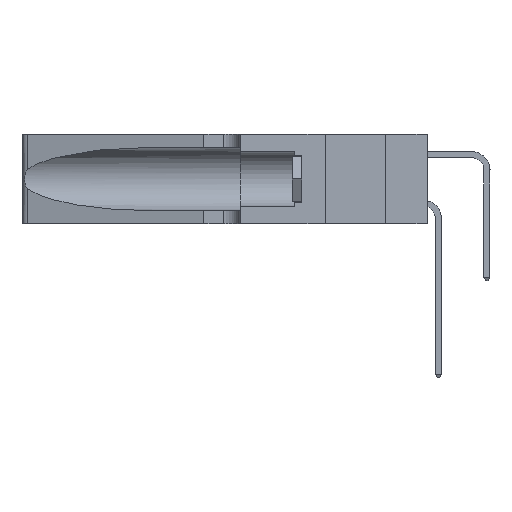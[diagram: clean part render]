
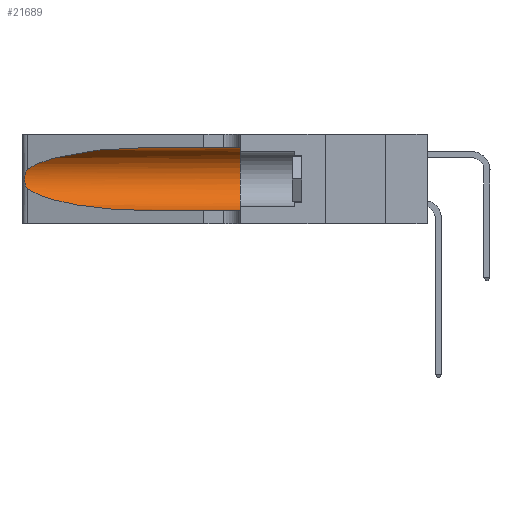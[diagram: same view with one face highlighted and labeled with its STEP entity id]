
A CAD part, left-side view. The second image highlights one B-rep face of the part: STEP entity #21689.
In plain terms, the highlighted cylindrical face has radius 3.308 mm (diameter 6.617 mm), a partial arc.
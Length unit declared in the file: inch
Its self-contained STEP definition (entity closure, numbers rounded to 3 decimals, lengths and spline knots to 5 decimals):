
#29 =( BOUNDED_CURVE ( )  B_SPLINE_CURVE ( 3, ( #14453, #12315, #16738, #3246 ),
 .UNSPECIFIED., .F., .T. ) 
 B_SPLINE_CURVE_WITH_KNOTS ( ( 4, 4 ),
 ( 1.5708, 2.84003 ),
 .UNSPECIFIED. ) 
 CURVE ( )  GEOMETRIC_REPRESENTATION_ITEM ( )  RATIONAL_B_SPLINE_CURVE ( ( 1., 0.87, 0.87, 1. ) ) 
 REPRESENTATION_ITEM ( '' )  );
#107 = VERTEX_POINT ( 'NONE', #23577 ) ;
#424 =( BOUNDED_CURVE ( )  B_SPLINE_CURVE ( 3, ( #24933, #11596, #27134, #13851 ),
 .UNSPECIFIED., .F., .F. ) 
 B_SPLINE_CURVE_WITH_KNOTS ( ( 4, 4 ),
 ( 3.44316, 4.71239 ),
 .UNSPECIFIED. ) 
 CURVE ( )  GEOMETRIC_REPRESENTATION_ITEM ( )  RATIONAL_B_SPLINE_CURVE ( ( 1., 0.87, 0.87, 1. ) ) 
 REPRESENTATION_ITEM ( '' )  );
#698 = VERTEX_POINT ( 'NONE', #26655 ) ;
#921 = CARTESIAN_POINT ( 'NONE',  ( 0.25639, 1.23184, 0.21858 ) ) ;
#1228 = ORIENTED_EDGE ( 'NONE', *, *, #6354, .T. ) ;
#2603 = ORIENTED_EDGE ( 'NONE', *, *, #28877, .T. ) ;
#2631 = CARTESIAN_POINT ( 'NONE',  ( 0.1305, 0.35, 0.05475 ) ) ;
#3054 = CARTESIAN_POINT ( 'NONE',  ( 0.1305, 1.61858, 0.185 ) ) ;
#3157 = DIRECTION ( 'NONE',  ( 0., -1., 0. ) ) ;
#3172 = CARTESIAN_POINT ( 'NONE',  ( 0.1305, 1.61858, 0.05475 ) ) ;
#3246 = CARTESIAN_POINT ( 'NONE',  ( 0.25487, 1.22718, 0.22369 ) ) ;
#3313 = CARTESIAN_POINT ( 'NONE',  ( 0.25854, 1.2359, 0.20912 ) ) ;
#3613 = EDGE_CURVE ( 'NONE', #698, #21969, #27777, .T. ) ;
#4062 = CARTESIAN_POINT ( 'NONE',  ( 0.1305, 0.35, 0.31525 ) ) ;
#4977 = CARTESIAN_POINT ( 'NONE',  ( 0.25487, 1.22718, 0.22369 ) ) ;
#5544 = DIRECTION ( 'NONE',  ( 0., -1., 0. ) ) ;
#5684 = CARTESIAN_POINT ( 'NONE',  ( 0.26075, 1.23896, 0.19203 ) ) ;
#6354 = EDGE_CURVE ( 'NONE', #21537, #107, #424, .T. ) ;
#6377 = DIRECTION ( 'NONE',  ( 0., -1., 0. ) ) ;
#6658 = AXIS2_PLACEMENT_3D ( 'NONE', #20485, #7155, #22737 ) ;
#7155 = DIRECTION ( 'NONE',  ( 0., 1., 0. ) ) ;
#7335 = CARTESIAN_POINT ( 'NONE',  ( 0.25487, 1.22718, 0.14631 ) ) ;
#7809 = EDGE_CURVE ( 'NONE', #698, #12076, #29, .T. ) ;
#7941 = CARTESIAN_POINT ( 'NONE',  ( 0.26017, 1.23833, 0.17102 ) ) ;
#10047 = VECTOR ( 'NONE', #6377, 39.37008 ) ;
#10084 = CARTESIAN_POINT ( 'NONE',  ( 0.25555, 1.22994, 0.2215 ) ) ;
#10189 = CARTESIAN_POINT ( 'NONE',  ( 0.25789, 1.23486, 0.15765 ) ) ;
#11387 = LINE ( 'NONE', #3172, #28360 ) ;
#11596 = CARTESIAN_POINT ( 'NONE',  ( 0.2373, 1.15595, 0.08982 ) ) ;
#11775 = EDGE_LOOP ( 'NONE', ( #20537, #16792, #1228, #2603, #23542, #26897 ) ) ;
#12076 = VERTEX_POINT ( 'NONE', #4977 ) ;
#12315 = CARTESIAN_POINT ( 'NONE',  ( 0.18966, 0.96281, 0.31525 ) ) ;
#12470 = CARTESIAN_POINT ( 'NONE',  ( 0.25555, 1.22993, 0.14849 ) ) ;
#13851 = CARTESIAN_POINT ( 'NONE',  ( 0.1305, 0.72297, 0.05475 ) ) ;
#14453 = CARTESIAN_POINT ( 'NONE',  ( 0.1305, 0.72297, 0.31525 ) ) ;
#15392 = EDGE_CURVE ( 'NONE', #12076, #21537, #23796, .T. ) ;
#16738 = CARTESIAN_POINT ( 'NONE',  ( 0.2373, 1.15595, 0.28018 ) ) ;
#16792 = ORIENTED_EDGE ( 'NONE', *, *, #15392, .T. ) ;
#16798 = CARTESIAN_POINT ( 'NONE',  ( 0.25787, 1.23484, 0.2124 ) ) ;
#17032 = CYLINDRICAL_SURFACE ( 'NONE', #28216, 0.13025 ) ;
#17701 = CIRCLE ( 'NONE', #6658, 0.13025 ) ;
#17721 = FACE_OUTER_BOUND ( 'NONE', #11775, .T. ) ;
#18868 = DIRECTION ( 'NONE',  ( 0., 0., -1. ) ) ;
#19017 = CARTESIAN_POINT ( 'NONE',  ( 0.26018, 1.23835, 0.19895 ) ) ;
#19203 = VERTEX_POINT ( 'NONE', #2631 ) ;
#19800 = CARTESIAN_POINT ( 'NONE',  ( 0.1305, 1.61858, 0.31525 ) ) ;
#20485 = CARTESIAN_POINT ( 'NONE',  ( 0.1305, 0.35, 0.185 ) ) ;
#20537 = ORIENTED_EDGE ( 'NONE', *, *, #7809, .T. ) ;
#21274 = CARTESIAN_POINT ( 'NONE',  ( 0.26075, 1.23896, 0.178 ) ) ;
#21537 = VERTEX_POINT ( 'NONE', #7335 ) ;
#21689 = ADVANCED_FACE ( 'NONE', ( #17721 ), #17032, .F. ) ;
#21969 = VERTEX_POINT ( 'NONE', #4062 ) ;
#22737 = DIRECTION ( 'NONE',  ( 0., 0., 1. ) ) ;
#22863 = EDGE_CURVE ( 'NONE', #21969, #19203, #17701, .T. ) ;
#23443 = CARTESIAN_POINT ( 'NONE',  ( 0.25487, 1.22718, 0.22369 ) ) ;
#23535 = CARTESIAN_POINT ( 'NONE',  ( 0.25856, 1.23593, 0.16098 ) ) ;
#23542 = ORIENTED_EDGE ( 'NONE', *, *, #22863, .F. ) ;
#23577 = CARTESIAN_POINT ( 'NONE',  ( 0.1305, 0.72297, 0.05475 ) ) ;
#23796 = B_SPLINE_CURVE_WITH_KNOTS ( 'NONE', 3,
 ( #23443, #10084, #921, #16798, #3313, #19017, #5684, #21274, #7941, #23535, #10189, #25761, #12470, #27945 ),
 .UNSPECIFIED., .F., .F.,
 ( 4, 2, 2, 2, 2, 2, 4 ),
 ( 0., 0.00027, 0.00053, 0.00107, 0.0016, 0.00187, 0.00214 ),
 .UNSPECIFIED. ) ;
#24933 = CARTESIAN_POINT ( 'NONE',  ( 0.25487, 1.22718, 0.14631 ) ) ;
#25761 = CARTESIAN_POINT ( 'NONE',  ( 0.25639, 1.23186, 0.15144 ) ) ;
#26655 = CARTESIAN_POINT ( 'NONE',  ( 0.1305, 0.72297, 0.31525 ) ) ;
#26897 = ORIENTED_EDGE ( 'NONE', *, *, #3613, .F. ) ;
#27134 = CARTESIAN_POINT ( 'NONE',  ( 0.18966, 0.96281, 0.05475 ) ) ;
#27777 = LINE ( 'NONE', #19800, #10047 ) ;
#27945 = CARTESIAN_POINT ( 'NONE',  ( 0.25487, 1.22718, 0.14631 ) ) ;
#28216 = AXIS2_PLACEMENT_3D ( 'NONE', #3054, #3157, #18868 ) ;
#28360 = VECTOR ( 'NONE', #5544, 39.37008 ) ;
#28877 = EDGE_CURVE ( 'NONE', #107, #19203, #11387, .T. ) ;
